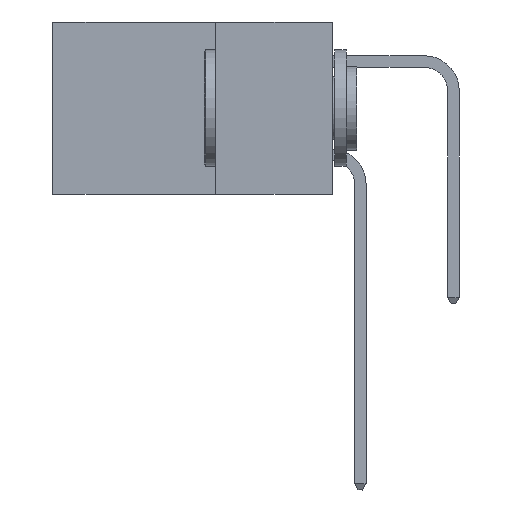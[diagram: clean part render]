
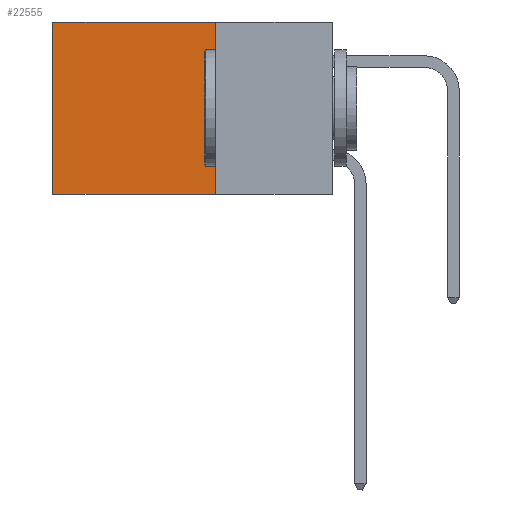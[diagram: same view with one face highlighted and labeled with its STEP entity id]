
A CAD part, left-side view. The second image highlights one B-rep face of the part: STEP entity #22555.
In plain terms, the highlighted planar face has unit normal (-1, 0, 0).
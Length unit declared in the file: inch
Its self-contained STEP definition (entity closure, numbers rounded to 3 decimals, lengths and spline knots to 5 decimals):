
#134 = CARTESIAN_POINT ( 'NONE',  ( 0.2615, 0.25, 0. ) ) ;
#1514 = ORIENTED_EDGE ( 'NONE', *, *, #2740, .F. ) ;
#2053 = DIRECTION ( 'NONE',  ( 0., 1., 0. ) ) ;
#2740 = EDGE_CURVE ( 'NONE', #2810, #11648, #7203, .T. ) ;
#2755 = CARTESIAN_POINT ( 'NONE',  ( 0.2615, 0.25, 0. ) ) ;
#2810 = VERTEX_POINT ( 'NONE', #2755 ) ;
#3009 = ORIENTED_EDGE ( 'NONE', *, *, #9534, .T. ) ;
#3106 = DIRECTION ( 'NONE',  ( 0., 1., 0. ) ) ;
#3485 = CARTESIAN_POINT ( 'NONE',  ( 0.2615, 0.6, -0.37 ) ) ;
#4940 = ORIENTED_EDGE ( 'NONE', *, *, #6680, .T. ) ;
#5078 = CARTESIAN_POINT ( 'NONE',  ( 0.2615, 0.25, -0.37 ) ) ;
#5278 = DIRECTION ( 'NONE',  ( 0., 0., -1. ) ) ;
#6680 = EDGE_CURVE ( 'NONE', #2810, #11962, #22558, .T. ) ;
#6949 = DIRECTION ( 'NONE',  ( 0., 0., -1. ) ) ;
#6982 = CARTESIAN_POINT ( 'NONE',  ( 0.2615, 0.25, -0.37 ) ) ;
#7151 = EDGE_LOOP ( 'NONE', ( #3009, #24475, #1514, #4940 ) ) ;
#7203 = LINE ( 'NONE', #6982, #11620 ) ;
#7965 = LINE ( 'NONE', #5078, #12371 ) ;
#8113 = CARTESIAN_POINT ( 'NONE',  ( 0.2615, 0.6, 0. ) ) ;
#9534 = EDGE_CURVE ( 'NONE', #11962, #19595, #23225, .T. ) ;
#10388 = DIRECTION ( 'NONE',  ( 0., 0., -1. ) ) ;
#10761 = EDGE_CURVE ( 'NONE', #11648, #19595, #7965, .T. ) ;
#11620 = VECTOR ( 'NONE', #5278, 39.37008 ) ;
#11648 = VERTEX_POINT ( 'NONE', #12909 ) ;
#11962 = VERTEX_POINT ( 'NONE', #8113 ) ;
#12371 = VECTOR ( 'NONE', #3106, 39.37008 ) ;
#12909 = CARTESIAN_POINT ( 'NONE',  ( 0.2615, 0.25, -0.37 ) ) ;
#16857 = VECTOR ( 'NONE', #2053, 39.37008 ) ;
#18115 = VECTOR ( 'NONE', #6949, 39.37008 ) ;
#19595 = VERTEX_POINT ( 'NONE', #3485 ) ;
#19893 = PLANE ( 'NONE',  #21115 ) ;
#20236 = CARTESIAN_POINT ( 'NONE',  ( 0.2615, 0.6, -0.37 ) ) ;
#21115 = AXIS2_PLACEMENT_3D ( 'NONE', #21744, #21823, #10388 ) ;
#21744 = CARTESIAN_POINT ( 'NONE',  ( 0.2615, 0.25, -0.37 ) ) ;
#21823 = DIRECTION ( 'NONE',  ( 1., 0., 0. ) ) ;
#21890 = FACE_OUTER_BOUND ( 'NONE', #7151, .T. ) ;
#22555 = ADVANCED_FACE ( 'NONE', ( #21890 ), #19893, .F. ) ;
#22558 = LINE ( 'NONE', #134, #16857 ) ;
#23225 = LINE ( 'NONE', #20236, #18115 ) ;
#24475 = ORIENTED_EDGE ( 'NONE', *, *, #10761, .F. ) ;
